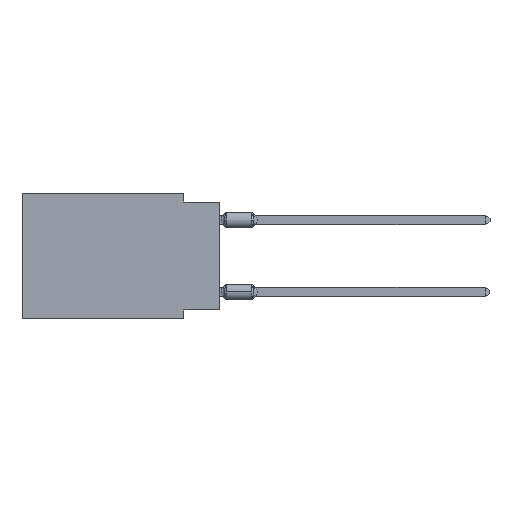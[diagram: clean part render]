
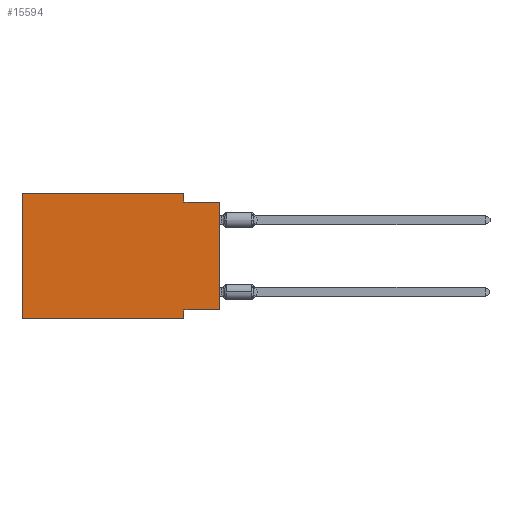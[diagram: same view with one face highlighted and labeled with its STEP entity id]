
A CAD part, left-side view. The second image highlights one B-rep face of the part: STEP entity #15594.
In plain terms, the highlighted planar face has unit normal (-1, 0, 0).
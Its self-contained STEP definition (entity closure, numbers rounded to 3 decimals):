
#119 = DIRECTION ( 'NONE',  ( 0., 0., 1. ) ) ;
#432 = DIRECTION ( 'NONE',  ( 0., 0., -1. ) ) ;
#778 = VERTEX_POINT ( 'NONE', #22658 ) ;
#924 = CARTESIAN_POINT ( 'NONE',  ( 0., 2.54, -8.89 ) ) ;
#943 = VECTOR ( 'NONE', #17724, 1000. ) ;
#1877 = DIRECTION ( 'NONE',  ( 0., 1., 0. ) ) ;
#1945 = VERTEX_POINT ( 'NONE', #3137 ) ;
#2600 = LINE ( 'NONE', #9487, #19281 ) ;
#3008 = CARTESIAN_POINT ( 'NONE',  ( 0., 13.97, -8.89 ) ) ;
#3137 = CARTESIAN_POINT ( 'NONE',  ( 0., 2.54, -8.255 ) ) ;
#3912 = CARTESIAN_POINT ( 'NONE',  ( 0., 0., -0.635 ) ) ;
#4052 = AXIS2_PLACEMENT_3D ( 'NONE', #5273, #21374, #432 ) ;
#4504 = ORIENTED_EDGE ( 'NONE', *, *, #6467, .F. ) ;
#4608 = VERTEX_POINT ( 'NONE', #3008 ) ;
#4678 = VECTOR ( 'NONE', #4689, 1000. ) ;
#4689 = DIRECTION ( 'NONE',  ( 0., -1., 0. ) ) ;
#5273 = CARTESIAN_POINT ( 'NONE',  ( 0., 13.97, 0. ) ) ;
#5419 = CARTESIAN_POINT ( 'NONE',  ( 0., 2.54, 0. ) ) ;
#5802 = ORIENTED_EDGE ( 'NONE', *, *, #19269, .F. ) ;
#5803 = DIRECTION ( 'NONE',  ( 0., 0., -1. ) ) ;
#6422 = LINE ( 'NONE', #13435, #4678 ) ;
#6467 = EDGE_CURVE ( 'NONE', #21593, #1945, #17304, .T. ) ;
#6579 = EDGE_CURVE ( 'NONE', #778, #13995, #10836, .T. ) ;
#7190 = VECTOR ( 'NONE', #13934, 1000. ) ;
#7473 = ORIENTED_EDGE ( 'NONE', *, *, #14117, .T. ) ;
#7746 = CARTESIAN_POINT ( 'NONE',  ( 0., 0., -0.635 ) ) ;
#7804 = EDGE_LOOP ( 'NONE', ( #7473, #17642, #16133, #5802, #12860, #9565, #17602, #4504 ) ) ;
#8016 = EDGE_CURVE ( 'NONE', #4608, #19905, #8762, .T. ) ;
#8083 = EDGE_CURVE ( 'NONE', #21730, #778, #10486, .T. ) ;
#8762 = LINE ( 'NONE', #12312, #7190 ) ;
#9130 = LINE ( 'NONE', #19830, #11344 ) ;
#9239 = CARTESIAN_POINT ( 'NONE',  ( 0., 13.97, 0. ) ) ;
#9487 = CARTESIAN_POINT ( 'NONE',  ( 0., 13.97, -8.89 ) ) ;
#9565 = ORIENTED_EDGE ( 'NONE', *, *, #16227, .T. ) ;
#9583 = VERTEX_POINT ( 'NONE', #924 ) ;
#10486 = LINE ( 'NONE', #5419, #943 ) ;
#10618 = CARTESIAN_POINT ( 'NONE',  ( 0., 0., -8.255 ) ) ;
#10836 = LINE ( 'NONE', #7746, #19944 ) ;
#11344 = VECTOR ( 'NONE', #5803, 1000. ) ;
#12025 = EDGE_CURVE ( 'NONE', #1945, #9583, #9130, .T. ) ;
#12303 = LINE ( 'NONE', #15867, #17619 ) ;
#12312 = CARTESIAN_POINT ( 'NONE',  ( 0., 13.97, 0. ) ) ;
#12860 = ORIENTED_EDGE ( 'NONE', *, *, #8016, .F. ) ;
#12897 = CARTESIAN_POINT ( 'NONE',  ( 0., 2.54, 0. ) ) ;
#13435 = CARTESIAN_POINT ( 'NONE',  ( 0., 13.97, 0. ) ) ;
#13934 = DIRECTION ( 'NONE',  ( 0., 0., 1. ) ) ;
#13995 = VERTEX_POINT ( 'NONE', #3912 ) ;
#14117 = EDGE_CURVE ( 'NONE', #21593, #13995, #12303, .T. ) ;
#14358 = FACE_OUTER_BOUND ( 'NONE', #7804, .T. ) ;
#15594 = ADVANCED_FACE ( 'NONE', ( #14358 ), #21143, .F. ) ;
#15867 = CARTESIAN_POINT ( 'NONE',  ( 0., 0., 0. ) ) ;
#16133 = ORIENTED_EDGE ( 'NONE', *, *, #8083, .F. ) ;
#16227 = EDGE_CURVE ( 'NONE', #4608, #9583, #2600, .T. ) ;
#17304 = LINE ( 'NONE', #19356, #18111 ) ;
#17602 = ORIENTED_EDGE ( 'NONE', *, *, #12025, .F. ) ;
#17619 = VECTOR ( 'NONE', #119, 1000. ) ;
#17642 = ORIENTED_EDGE ( 'NONE', *, *, #6579, .F. ) ;
#17724 = DIRECTION ( 'NONE',  ( 0., 0., -1. ) ) ;
#18111 = VECTOR ( 'NONE', #1877, 1000. ) ;
#18121 = DIRECTION ( 'NONE',  ( 0., -1., 0. ) ) ;
#19269 = EDGE_CURVE ( 'NONE', #19905, #21730, #6422, .T. ) ;
#19281 = VECTOR ( 'NONE', #18121, 1000. ) ;
#19356 = CARTESIAN_POINT ( 'NONE',  ( 0., 0., -8.255 ) ) ;
#19698 = DIRECTION ( 'NONE',  ( 0., -1., 0. ) ) ;
#19830 = CARTESIAN_POINT ( 'NONE',  ( 0., 2.54, -8.89 ) ) ;
#19905 = VERTEX_POINT ( 'NONE', #9239 ) ;
#19944 = VECTOR ( 'NONE', #19698, 1000. ) ;
#21143 = PLANE ( 'NONE',  #4052 ) ;
#21374 = DIRECTION ( 'NONE',  ( 1., 0., 0. ) ) ;
#21593 = VERTEX_POINT ( 'NONE', #10618 ) ;
#21730 = VERTEX_POINT ( 'NONE', #12897 ) ;
#22658 = CARTESIAN_POINT ( 'NONE',  ( 0., 2.54, -0.635 ) ) ;
